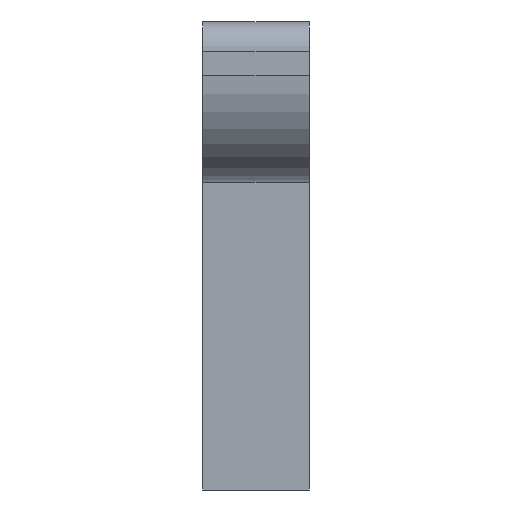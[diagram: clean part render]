
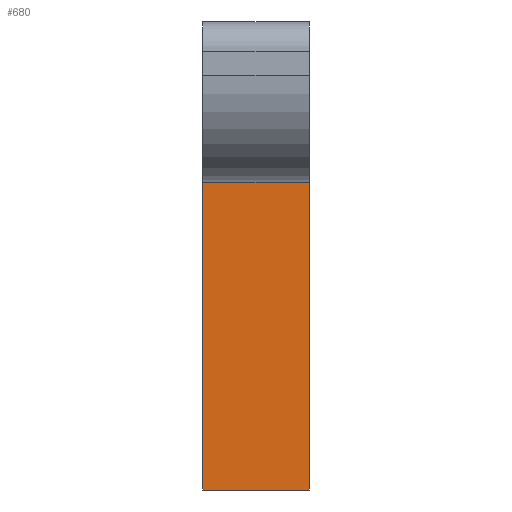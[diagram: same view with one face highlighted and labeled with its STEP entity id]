
A CAD part, front view. The second image highlights one B-rep face of the part: STEP entity #680.
In plain terms, the highlighted planar face has unit normal (0, -1, 0).
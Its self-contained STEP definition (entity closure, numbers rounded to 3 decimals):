
#8 = DIRECTION ( 'NONE',  ( -1., 0., 0. ) ) ;
#64 = LINE ( 'NONE', #283, #271 ) ;
#65 = VECTOR ( 'NONE', #285, 1000. ) ;
#105 = EDGE_CURVE ( 'NONE', #248, #880, #628, .T. ) ;
#107 = ORIENTED_EDGE ( 'NONE', *, *, #239, .F. ) ;
#167 = DIRECTION ( 'NONE',  ( 0., 0., 1. ) ) ;
#172 = CARTESIAN_POINT ( 'NONE',  ( 10., -5.181, 12.462 ) ) ;
#173 = VECTOR ( 'NONE', #8, 1000. ) ;
#175 = ORIENTED_EDGE ( 'NONE', *, *, #869, .F. ) ;
#179 = VERTEX_POINT ( 'NONE', #670 ) ;
#182 = ORIENTED_EDGE ( 'NONE', *, *, #105, .T. ) ;
#234 = CARTESIAN_POINT ( 'NONE',  ( 10., -5.181, -26.402 ) ) ;
#239 = EDGE_CURVE ( 'NONE', #622, #880, #895, .T. ) ;
#247 = LINE ( 'NONE', #630, #65 ) ;
#248 = VERTEX_POINT ( 'NONE', #625 ) ;
#260 = VECTOR ( 'NONE', #802, 1000. ) ;
#271 = VECTOR ( 'NONE', #292, 1000. ) ;
#283 = CARTESIAN_POINT ( 'NONE',  ( 10., -5.181, 2.462 ) ) ;
#285 = DIRECTION ( 'NONE',  ( 0., 0., -1. ) ) ;
#292 = DIRECTION ( 'NONE',  ( 1., 0., 0. ) ) ;
#382 = EDGE_CURVE ( 'NONE', #179, #622, #247, .T. ) ;
#386 = DIRECTION ( 'NONE',  ( 0., 1., 0. ) ) ;
#527 = PLANE ( 'NONE',  #572 ) ;
#563 = FACE_OUTER_BOUND ( 'NONE', #642, .T. ) ;
#572 = AXIS2_PLACEMENT_3D ( 'NONE', #172, #386, #167 ) ;
#622 = VERTEX_POINT ( 'NONE', #694 ) ;
#625 = CARTESIAN_POINT ( 'NONE',  ( 0., -5.181, 2.462 ) ) ;
#628 = LINE ( 'NONE', #674, #260 ) ;
#630 = CARTESIAN_POINT ( 'NONE',  ( 10., -5.181, 12.462 ) ) ;
#642 = EDGE_LOOP ( 'NONE', ( #175, #182, #107, #801 ) ) ;
#670 = CARTESIAN_POINT ( 'NONE',  ( 10., -5.181, 2.462 ) ) ;
#674 = CARTESIAN_POINT ( 'NONE',  ( 0., -5.181, 12.462 ) ) ;
#680 = ADVANCED_FACE ( 'NONE', ( #563 ), #527, .F. ) ;
#694 = CARTESIAN_POINT ( 'NONE',  ( 10., -5.181, -26.402 ) ) ;
#800 = CARTESIAN_POINT ( 'NONE',  ( 0., -5.181, -26.402 ) ) ;
#801 = ORIENTED_EDGE ( 'NONE', *, *, #382, .F. ) ;
#802 = DIRECTION ( 'NONE',  ( 0., 0., -1. ) ) ;
#869 = EDGE_CURVE ( 'NONE', #248, #179, #64, .T. ) ;
#880 = VERTEX_POINT ( 'NONE', #800 ) ;
#895 = LINE ( 'NONE', #234, #173 ) ;
